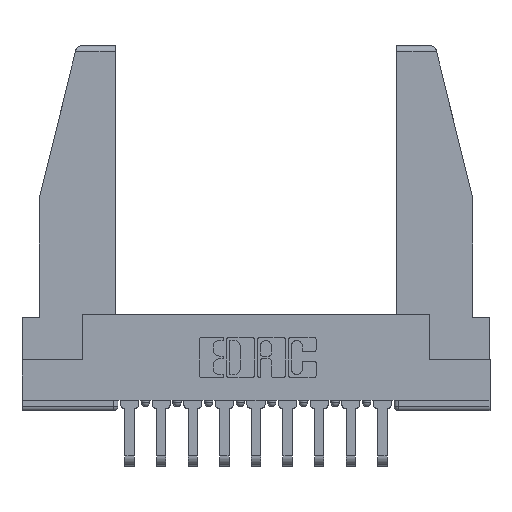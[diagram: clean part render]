
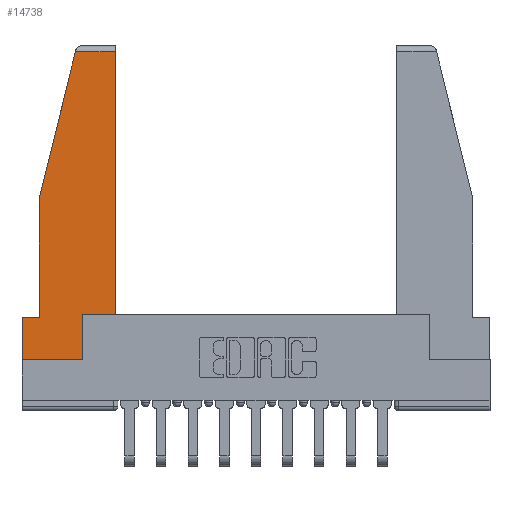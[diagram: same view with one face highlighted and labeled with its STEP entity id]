
A CAD part, top view. The second image highlights one B-rep face of the part: STEP entity #14738.
In plain terms, the highlighted planar face has unit normal (0, 0, 1).
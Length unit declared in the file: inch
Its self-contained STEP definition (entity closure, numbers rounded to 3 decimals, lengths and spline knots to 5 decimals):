
#70 = CARTESIAN_POINT ( 'NONE',  ( 0.2636, 1.52, 0. ) ) ;
#211 = DIRECTION ( 'NONE',  ( 0., 1., 0. ) ) ;
#778 = DIRECTION ( 'NONE',  ( -0.239, -0.971, 0. ) ) ;
#812 = EDGE_LOOP ( 'NONE', ( #5765, #6044, #8754, #3427, #14758, #3889, #12234, #14136, #13095 ) ) ;
#819 = CARTESIAN_POINT ( 'NONE',  ( 0.297, 0.223, 0. ) ) ;
#872 = DIRECTION ( 'NONE',  ( 1., 0., 0. ) ) ;
#1219 = CARTESIAN_POINT ( 'NONE',  ( 0., 0.21, 0. ) ) ;
#1245 = VECTOR ( 'NONE', #7524, 39.37008 ) ;
#1287 = CARTESIAN_POINT ( 'NONE',  ( 0.461, 0.223, 0. ) ) ;
#1723 = CARTESIAN_POINT ( 'NONE',  ( 0., 0., 0. ) ) ;
#2097 = AXIS2_PLACEMENT_3D ( 'NONE', #12179, #15939, #8555 ) ;
#2280 = VERTEX_POINT ( 'NONE', #9874 ) ;
#2591 = DIRECTION ( 'NONE',  ( 0., 1., 0. ) ) ;
#2592 = LINE ( 'NONE', #1219, #1245 ) ;
#2618 = CARTESIAN_POINT ( 'NONE',  ( 0., 0.21, 0. ) ) ;
#2690 = LINE ( 'NONE', #4598, #9244 ) ;
#3158 = VECTOR ( 'NONE', #872, 39.37008 ) ;
#3219 = CARTESIAN_POINT ( 'NONE',  ( 0.297, 0., 0. ) ) ;
#3427 = ORIENTED_EDGE ( 'NONE', *, *, #4699, .T. ) ;
#3690 = VECTOR ( 'NONE', #11264, 39.37008 ) ;
#3889 = ORIENTED_EDGE ( 'NONE', *, *, #12454, .T. ) ;
#4090 = CARTESIAN_POINT ( 'NONE',  ( 0.461, 1.52, 0. ) ) ;
#4292 = VERTEX_POINT ( 'NONE', #70 ) ;
#4577 = VERTEX_POINT ( 'NONE', #1723 ) ;
#4598 = CARTESIAN_POINT ( 'NONE',  ( 0., 1.52, 0. ) ) ;
#4699 = EDGE_CURVE ( 'NONE', #5804, #2280, #10996, .T. ) ;
#4781 = EDGE_CURVE ( 'NONE', #14243, #4292, #2690, .T. ) ;
#4911 = VECTOR ( 'NONE', #778, 39.37008 ) ;
#5588 = VECTOR ( 'NONE', #9350, 39.37008 ) ;
#5683 = CARTESIAN_POINT ( 'NONE',  ( 0.086, 0.8, 0. ) ) ;
#5686 = DIRECTION ( 'NONE',  ( -1., 0., 0. ) ) ;
#5747 = CARTESIAN_POINT ( 'NONE',  ( 0.297, 0., 0. ) ) ;
#5765 = ORIENTED_EDGE ( 'NONE', *, *, #14090, .T. ) ;
#5804 = VERTEX_POINT ( 'NONE', #5683 ) ;
#6044 = ORIENTED_EDGE ( 'NONE', *, *, #4781, .T. ) ;
#6879 = CARTESIAN_POINT ( 'NONE',  ( 0.271, 1.55, 0. ) ) ;
#7387 = VECTOR ( 'NONE', #2591, 39.37008 ) ;
#7524 = DIRECTION ( 'NONE',  ( 0., -1., 0. ) ) ;
#7549 = FACE_OUTER_BOUND ( 'NONE', #812, .T. ) ;
#7969 = LINE ( 'NONE', #15368, #3158 ) ;
#8038 = EDGE_CURVE ( 'NONE', #4292, #5804, #10696, .T. ) ;
#8555 = DIRECTION ( 'NONE',  ( 1., 0., 0. ) ) ;
#8754 = ORIENTED_EDGE ( 'NONE', *, *, #8038, .T. ) ;
#9166 = CARTESIAN_POINT ( 'NONE',  ( 0.461, 0.223, 0. ) ) ;
#9244 = VECTOR ( 'NONE', #5686, 39.37008 ) ;
#9302 = VERTEX_POINT ( 'NONE', #9166 ) ;
#9350 = DIRECTION ( 'NONE',  ( 0., -1., 0. ) ) ;
#9850 = LINE ( 'NONE', #2618, #3690 ) ;
#9874 = CARTESIAN_POINT ( 'NONE',  ( 0.086, 0.21, 0. ) ) ;
#9923 = LINE ( 'NONE', #5747, #12989 ) ;
#9978 = EDGE_CURVE ( 'NONE', #10523, #9302, #13329, .T. ) ;
#10286 = EDGE_CURVE ( 'NONE', #2280, #13382, #9850, .T. ) ;
#10523 = VERTEX_POINT ( 'NONE', #819 ) ;
#10696 = LINE ( 'NONE', #6879, #4911 ) ;
#10996 = LINE ( 'NONE', #15427, #5588 ) ;
#11264 = DIRECTION ( 'NONE',  ( -1., 0., 0. ) ) ;
#11276 = LINE ( 'NONE', #1287, #7387 ) ;
#11595 = VECTOR ( 'NONE', #15391, 39.37008 ) ;
#12179 = CARTESIAN_POINT ( 'NONE',  ( 0., 0., 0. ) ) ;
#12234 = ORIENTED_EDGE ( 'NONE', *, *, #13800, .T. ) ;
#12454 = EDGE_CURVE ( 'NONE', #13382, #4577, #2592, .T. ) ;
#12812 = VERTEX_POINT ( 'NONE', #3219 ) ;
#12989 = VECTOR ( 'NONE', #211, 39.37008 ) ;
#12990 = EDGE_CURVE ( 'NONE', #12812, #10523, #9923, .T. ) ;
#13095 = ORIENTED_EDGE ( 'NONE', *, *, #9978, .T. ) ;
#13329 = LINE ( 'NONE', #15557, #11595 ) ;
#13340 = CARTESIAN_POINT ( 'NONE',  ( 0., 0.21, 0. ) ) ;
#13382 = VERTEX_POINT ( 'NONE', #13340 ) ;
#13800 = EDGE_CURVE ( 'NONE', #4577, #12812, #7969, .T. ) ;
#14090 = EDGE_CURVE ( 'NONE', #9302, #14243, #11276, .T. ) ;
#14136 = ORIENTED_EDGE ( 'NONE', *, *, #12990, .T. ) ;
#14243 = VERTEX_POINT ( 'NONE', #4090 ) ;
#14697 = PLANE ( 'NONE',  #2097 ) ;
#14738 = ADVANCED_FACE ( 'NONE', ( #7549 ), #14697, .T. ) ;
#14758 = ORIENTED_EDGE ( 'NONE', *, *, #10286, .T. ) ;
#15368 = CARTESIAN_POINT ( 'NONE',  ( 0., 0., 0. ) ) ;
#15391 = DIRECTION ( 'NONE',  ( 1., 0., 0. ) ) ;
#15427 = CARTESIAN_POINT ( 'NONE',  ( 0.086, 0.8, 0. ) ) ;
#15557 = CARTESIAN_POINT ( 'NONE',  ( 0.297, 0.223, 0. ) ) ;
#15939 = DIRECTION ( 'NONE',  ( 0., 0., 1. ) ) ;
